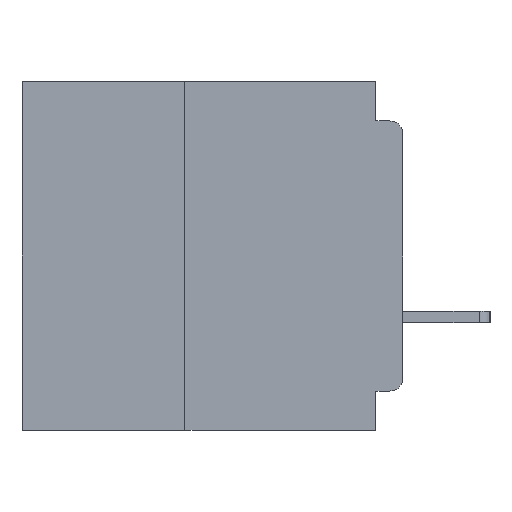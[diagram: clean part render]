
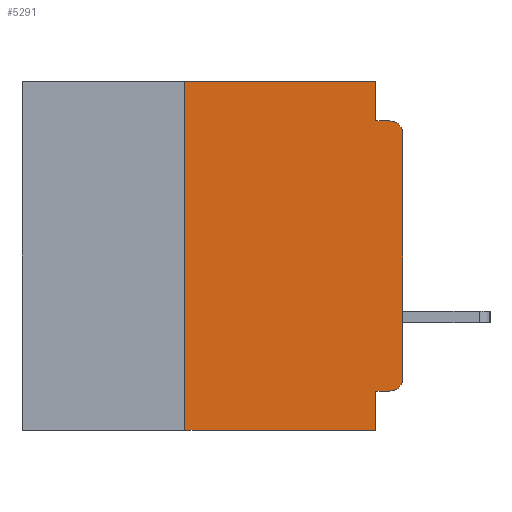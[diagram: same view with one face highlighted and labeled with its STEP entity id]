
A CAD part, left-side view. The second image highlights one B-rep face of the part: STEP entity #5291.
In plain terms, the highlighted planar face has unit normal (-1, 0, 0).
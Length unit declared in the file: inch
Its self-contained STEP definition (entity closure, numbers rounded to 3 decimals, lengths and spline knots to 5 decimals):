
#19 = ORIENTED_EDGE ( 'NONE', *, *, #27264, .F. ) ;
#618 = CARTESIAN_POINT ( 'NONE',  ( 0., 0.25, 0. ) ) ;
#1052 = CARTESIAN_POINT ( 'NONE',  ( 0., 0., -0.34 ) ) ;
#1791 = CARTESIAN_POINT ( 'NONE',  ( 0., 0.015, -0.06 ) ) ;
#3080 = VERTEX_POINT ( 'NONE', #9635 ) ;
#3623 = EDGE_CURVE ( 'NONE', #11059, #28660, #39636, .T. ) ;
#4093 = EDGE_CURVE ( 'NONE', #22335, #31076, #36709, .T. ) ;
#4300 = ORIENTED_EDGE ( 'NONE', *, *, #10064, .F. ) ;
#4420 = ORIENTED_EDGE ( 'NONE', *, *, #16254, .T. ) ;
#4809 = ORIENTED_EDGE ( 'NONE', *, *, #3623, .T. ) ;
#5090 = DIRECTION ( 'NONE',  ( 0., 0., -1. ) ) ;
#5291 = ADVANCED_FACE ( 'NONE', ( #12072 ), #36436, .F. ) ;
#5336 = AXIS2_PLACEMENT_3D ( 'NONE', #34607, #15661, #37743 ) ;
#5481 = VECTOR ( 'NONE', #36217, 39.37008 ) ;
#5592 = DIRECTION ( 'NONE',  ( 0., -1., 0. ) ) ;
#6394 = DIRECTION ( 'NONE',  ( 0., 0., -1. ) ) ;
#6402 = LINE ( 'NONE', #38071, #22513 ) ;
#6433 = ORIENTED_EDGE ( 'NONE', *, *, #35598, .F. ) ;
#7192 = LINE ( 'NONE', #23264, #23271 ) ;
#7261 = DIRECTION ( 'NONE',  ( 0., 0., 1. ) ) ;
#7800 = CARTESIAN_POINT ( 'NONE',  ( 0., 0.437, 0. ) ) ;
#9635 = CARTESIAN_POINT ( 'NONE',  ( 0., 0., -0.06 ) ) ;
#10064 = EDGE_CURVE ( 'NONE', #36306, #25668, #19740, .T. ) ;
#11059 = VERTEX_POINT ( 'NONE', #16743 ) ;
#11340 = CARTESIAN_POINT ( 'NONE',  ( 0., 0.031, 0. ) ) ;
#11378 = ORIENTED_EDGE ( 'NONE', *, *, #26720, .F. ) ;
#11457 = ORIENTED_EDGE ( 'NONE', *, *, #20158, .T. ) ;
#11601 = VECTOR ( 'NONE', #38513, 39.37008 ) ;
#12072 = FACE_OUTER_BOUND ( 'NONE', #13233, .T. ) ;
#12599 = LINE ( 'NONE', #29157, #11601 ) ;
#12881 = CARTESIAN_POINT ( 'NONE',  ( 0., 0.015, -0.045 ) ) ;
#13233 = EDGE_LOOP ( 'NONE', ( #4420, #11457, #37929, #4300, #19, #6433, #13452, #24259, #11378, #4809 ) ) ;
#13452 = ORIENTED_EDGE ( 'NONE', *, *, #4093, .T. ) ;
#14095 = CARTESIAN_POINT ( 'NONE',  ( 0., 0., 0. ) ) ;
#14545 = DIRECTION ( 'NONE',  ( 0., 0., -1. ) ) ;
#15661 = DIRECTION ( 'NONE',  ( -1., 0., 0. ) ) ;
#16254 = EDGE_CURVE ( 'NONE', #28660, #3080, #22607, .T. ) ;
#16743 = CARTESIAN_POINT ( 'NONE',  ( 0., 0.015, -0.355 ) ) ;
#17952 = VERTEX_POINT ( 'NONE', #618 ) ;
#18711 = VECTOR ( 'NONE', #14545, 39.37008 ) ;
#19740 = LINE ( 'NONE', #11340, #18711 ) ;
#19957 = VECTOR ( 'NONE', #5592, 39.37008 ) ;
#20158 = EDGE_CURVE ( 'NONE', #3080, #23586, #22547, .T. ) ;
#20733 = DIRECTION ( 'NONE',  ( 0., 0., -1. ) ) ;
#21623 = CARTESIAN_POINT ( 'NONE',  ( 0., 0.437, -0.4 ) ) ;
#22335 = VERTEX_POINT ( 'NONE', #41084 ) ;
#22513 = VECTOR ( 'NONE', #6394, 39.37008 ) ;
#22547 = CIRCLE ( 'NONE', #37777, 0.015 ) ;
#22607 = LINE ( 'NONE', #14095, #5481 ) ;
#22987 = CARTESIAN_POINT ( 'NONE',  ( 0., 0.437, 0. ) ) ;
#23119 = EDGE_CURVE ( 'NONE', #25668, #23586, #7192, .T. ) ;
#23264 = CARTESIAN_POINT ( 'NONE',  ( 0., 0., -0.045 ) ) ;
#23271 = VECTOR ( 'NONE', #26455, 39.37008 ) ;
#23586 = VERTEX_POINT ( 'NONE', #12881 ) ;
#24259 = ORIENTED_EDGE ( 'NONE', *, *, #27753, .F. ) ;
#24338 = DIRECTION ( 'NONE',  ( -1., 0., 0. ) ) ;
#24737 = CARTESIAN_POINT ( 'NONE',  ( 0., 0.031, -0.4 ) ) ;
#25668 = VERTEX_POINT ( 'NONE', #39386 ) ;
#26418 = CARTESIAN_POINT ( 'NONE',  ( 0., 0.031, -0.355 ) ) ;
#26455 = DIRECTION ( 'NONE',  ( 0., -1., 0. ) ) ;
#26720 = EDGE_CURVE ( 'NONE', #11059, #30799, #12599, .T. ) ;
#27264 = EDGE_CURVE ( 'NONE', #17952, #36306, #40152, .T. ) ;
#27753 = EDGE_CURVE ( 'NONE', #30799, #31076, #6402, .T. ) ;
#28660 = VERTEX_POINT ( 'NONE', #1052 ) ;
#29157 = CARTESIAN_POINT ( 'NONE',  ( 0., 0., -0.355 ) ) ;
#29257 = DIRECTION ( 'NONE',  ( 0., -1., 0. ) ) ;
#30799 = VERTEX_POINT ( 'NONE', #26418 ) ;
#31076 = VERTEX_POINT ( 'NONE', #24737 ) ;
#32063 = VECTOR ( 'NONE', #7261, 39.37008 ) ;
#32608 = CARTESIAN_POINT ( 'NONE',  ( 0., 0.031, 0. ) ) ;
#33035 = LINE ( 'NONE', #39003, #32063 ) ;
#34607 = CARTESIAN_POINT ( 'NONE',  ( 0., 0.015, -0.34 ) ) ;
#35598 = EDGE_CURVE ( 'NONE', #22335, #17952, #33035, .T. ) ;
#36217 = DIRECTION ( 'NONE',  ( 0., 0., 1. ) ) ;
#36306 = VERTEX_POINT ( 'NONE', #32608 ) ;
#36333 = AXIS2_PLACEMENT_3D ( 'NONE', #7800, #39517, #20733 ) ;
#36436 = PLANE ( 'NONE',  #36333 ) ;
#36709 = LINE ( 'NONE', #21623, #19957 ) ;
#37743 = DIRECTION ( 'NONE',  ( 0., 0., -1. ) ) ;
#37777 = AXIS2_PLACEMENT_3D ( 'NONE', #1791, #24338, #5090 ) ;
#37929 = ORIENTED_EDGE ( 'NONE', *, *, #23119, .F. ) ;
#38071 = CARTESIAN_POINT ( 'NONE',  ( 0., 0.031, -0.4 ) ) ;
#38513 = DIRECTION ( 'NONE',  ( 0., 1., 0. ) ) ;
#39003 = CARTESIAN_POINT ( 'NONE',  ( 0., 0.25, -0.4 ) ) ;
#39203 = VECTOR ( 'NONE', #29257, 39.37008 ) ;
#39386 = CARTESIAN_POINT ( 'NONE',  ( 0., 0.031, -0.045 ) ) ;
#39517 = DIRECTION ( 'NONE',  ( 1., 0., 0. ) ) ;
#39636 = CIRCLE ( 'NONE', #5336, 0.015 ) ;
#40152 = LINE ( 'NONE', #22987, #39203 ) ;
#41084 = CARTESIAN_POINT ( 'NONE',  ( 0., 0.25, -0.4 ) ) ;
